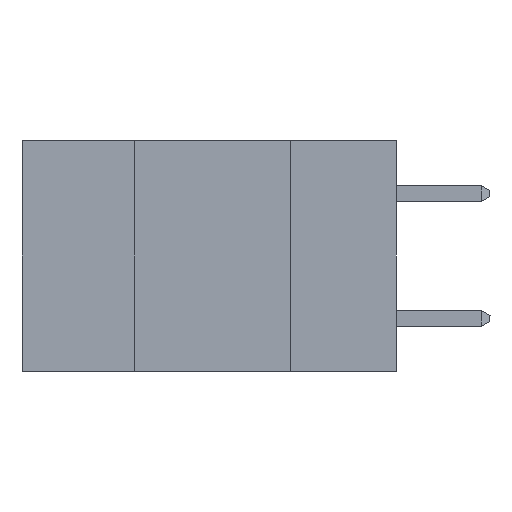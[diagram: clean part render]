
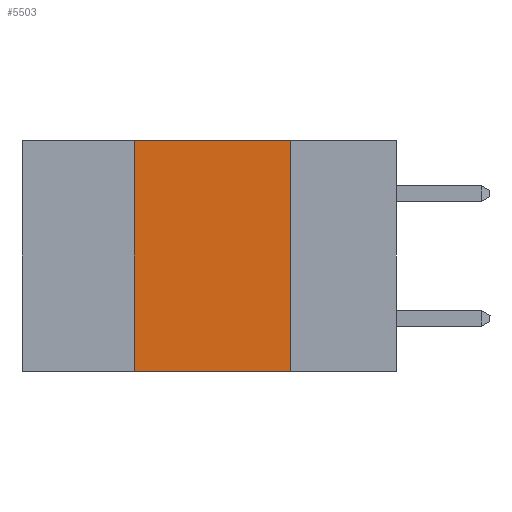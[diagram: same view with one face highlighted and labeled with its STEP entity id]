
A CAD part, left-side view. The second image highlights one B-rep face of the part: STEP entity #5503.
In plain terms, the highlighted planar face has unit normal (-1, 0, 0).
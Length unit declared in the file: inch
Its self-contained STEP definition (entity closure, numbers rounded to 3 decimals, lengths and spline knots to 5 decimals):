
#507 = LINE ( 'NONE', #14638, #13807 ) ;
#768 = CARTESIAN_POINT ( 'NONE',  ( 0., 0.17, -0.37 ) ) ;
#863 = LINE ( 'NONE', #20335, #18635 ) ;
#1662 = EDGE_CURVE ( 'NONE', #13292, #7835, #507, .T. ) ;
#1685 = ORIENTED_EDGE ( 'NONE', *, *, #1662, .F. ) ;
#2196 = CARTESIAN_POINT ( 'NONE',  ( 0., 0.17, -0.37 ) ) ;
#2843 = EDGE_CURVE ( 'NONE', #4237, #13292, #10809, .T. ) ;
#3242 = DIRECTION ( 'NONE',  ( 0., 0., -1. ) ) ;
#3995 = VECTOR ( 'NONE', #4000, 39.37008 ) ;
#4000 = DIRECTION ( 'NONE',  ( 0., 0., -1. ) ) ;
#4237 = VERTEX_POINT ( 'NONE', #16973 ) ;
#4570 = LINE ( 'NONE', #2196, #3995 ) ;
#5163 = DIRECTION ( 'NONE',  ( 0., -1., 0. ) ) ;
#5503 = ADVANCED_FACE ( 'NONE', ( #8634 ), #21933, .F. ) ;
#5720 = VECTOR ( 'NONE', #10175, 39.37008 ) ;
#7258 = EDGE_LOOP ( 'NONE', ( #14867, #1685, #20420, #20950 ) ) ;
#7835 = VERTEX_POINT ( 'NONE', #15368 ) ;
#8634 = FACE_OUTER_BOUND ( 'NONE', #7258, .T. ) ;
#9022 = EDGE_CURVE ( 'NONE', #4237, #17557, #863, .T. ) ;
#10005 = CARTESIAN_POINT ( 'NONE',  ( 0., 0.42, -0.37 ) ) ;
#10175 = DIRECTION ( 'NONE',  ( 0., 0., 1. ) ) ;
#10809 = LINE ( 'NONE', #10005, #5720 ) ;
#11846 = CARTESIAN_POINT ( 'NONE',  ( 0., 0.6, 0. ) ) ;
#13155 = AXIS2_PLACEMENT_3D ( 'NONE', #11846, #13538, #3242 ) ;
#13292 = VERTEX_POINT ( 'NONE', #19425 ) ;
#13538 = DIRECTION ( 'NONE',  ( 1., 0., 0. ) ) ;
#13807 = VECTOR ( 'NONE', #15391, 39.37008 ) ;
#14638 = CARTESIAN_POINT ( 'NONE',  ( 0., 0.6, 0. ) ) ;
#14867 = ORIENTED_EDGE ( 'NONE', *, *, #21548, .F. ) ;
#15368 = CARTESIAN_POINT ( 'NONE',  ( 0., 0.17, 0. ) ) ;
#15391 = DIRECTION ( 'NONE',  ( 0., -1., 0. ) ) ;
#16973 = CARTESIAN_POINT ( 'NONE',  ( 0., 0.42, -0.37 ) ) ;
#17557 = VERTEX_POINT ( 'NONE', #768 ) ;
#18635 = VECTOR ( 'NONE', #5163, 39.37008 ) ;
#19425 = CARTESIAN_POINT ( 'NONE',  ( 0., 0.42, 0. ) ) ;
#20335 = CARTESIAN_POINT ( 'NONE',  ( 0., 0.6, -0.37 ) ) ;
#20420 = ORIENTED_EDGE ( 'NONE', *, *, #2843, .F. ) ;
#20950 = ORIENTED_EDGE ( 'NONE', *, *, #9022, .T. ) ;
#21548 = EDGE_CURVE ( 'NONE', #7835, #17557, #4570, .T. ) ;
#21933 = PLANE ( 'NONE',  #13155 ) ;
